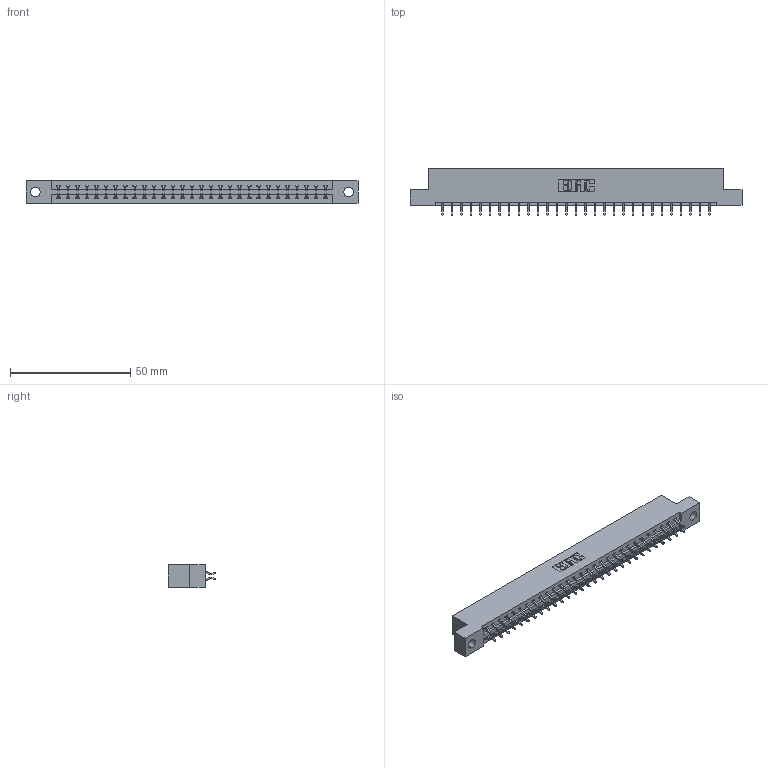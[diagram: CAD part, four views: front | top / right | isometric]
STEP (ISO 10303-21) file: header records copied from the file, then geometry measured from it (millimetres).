
FILE_DESCRIPTION (( 'STEP AP203' ), '1' );
FILE_NAME ('337-058-556-204.STEP', '2019-10-09T19:57:22', ( '' ), ( '' ), 'SwSTEP 2.0', 'SolidWorks 2016', '' );
FILE_SCHEMA (( 'CONFIG_CONTROL_DESIGN' ));
Length unit declared in the file: inch
Products named in the file (3): 345-292-001_556 Tail; 337 Part_Flush Mounting Lugs - 0.156 Dia-TH; 337-058-556-204
Assembly tree (59 placements, depth 2):
  337-058-556-204
    337 Part_Flush Mounting Lugs - 0.156 Dia-TH
    345-292-001_556 Tail  x58
Bounding box: 137.92 x 19.57 x 9.4 mm (x, y, z)
Volume: 14272.1 mm3; surface area: 15744.6 mm2
Topology: 59 solids, 59 shells, 3594 faces, 10693 edges, 7050 vertices
Faces by surface type: plane 2506, cylinder 1088
Entity records: 24389 total; most frequent: CARTESIAN_POINT 4134, ORIENTED_EDGE 4058, DIRECTION 3529, EDGE_CURVE 2029, VECTOR 1893, LINE 1893, VERTEX_POINT 1350, AXIS2_PLACEMENT_3D 818
